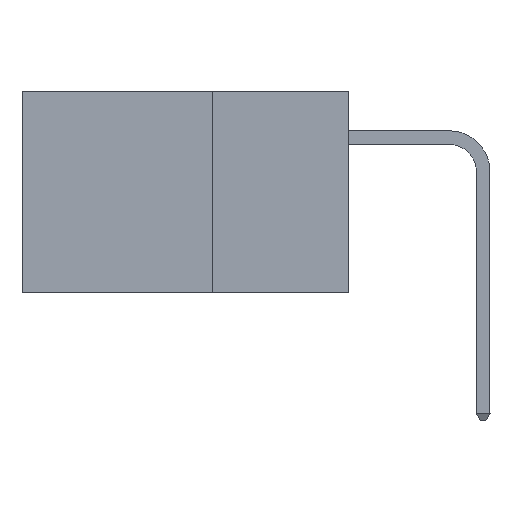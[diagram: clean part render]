
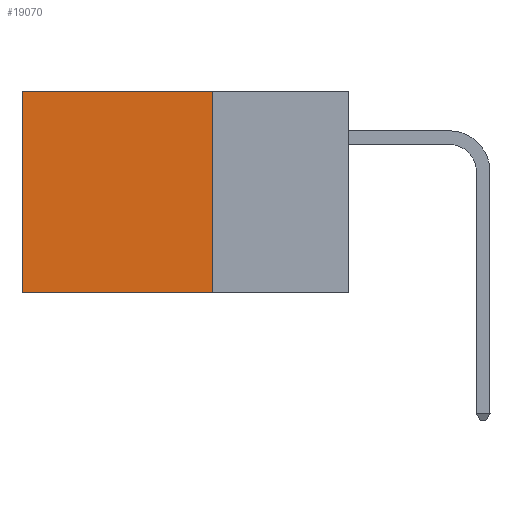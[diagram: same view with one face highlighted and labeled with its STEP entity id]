
A CAD part, left-side view. The second image highlights one B-rep face of the part: STEP entity #19070.
In plain terms, the highlighted planar face has unit normal (-1, 0, 0).
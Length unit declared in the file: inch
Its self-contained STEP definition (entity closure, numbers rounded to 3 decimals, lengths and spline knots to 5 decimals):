
#576 = EDGE_CURVE ( 'NONE', #24592, #1277, #18987, .T. ) ;
#1277 = VERTEX_POINT ( 'NONE', #18272 ) ;
#1332 = ORIENTED_EDGE ( 'NONE', *, *, #10872, .F. ) ;
#1830 = CARTESIAN_POINT ( 'NONE',  ( 0.2875, 0.25, 0. ) ) ;
#2749 = CARTESIAN_POINT ( 'NONE',  ( 0.2875, 0.6, 0. ) ) ;
#3491 = LINE ( 'NONE', #5325, #19199 ) ;
#5055 = VECTOR ( 'NONE', #14273, 39.37008 ) ;
#5325 = CARTESIAN_POINT ( 'NONE',  ( 0.2875, 0.25, -0.37 ) ) ;
#5871 = AXIS2_PLACEMENT_3D ( 'NONE', #6018, #14268, #10321 ) ;
#6018 = CARTESIAN_POINT ( 'NONE',  ( 0.2875, 0.25, 0. ) ) ;
#6700 = EDGE_CURVE ( 'NONE', #17373, #1277, #3491, .T. ) ;
#7690 = VERTEX_POINT ( 'NONE', #10959 ) ;
#8806 = CARTESIAN_POINT ( 'NONE',  ( 0.2875, 0.25, -0.37 ) ) ;
#10049 = CARTESIAN_POINT ( 'NONE',  ( 0.2875, 0.6, 0. ) ) ;
#10321 = DIRECTION ( 'NONE',  ( 0., 0., -1. ) ) ;
#10474 = EDGE_CURVE ( 'NONE', #7690, #24592, #12975, .T. ) ;
#10872 = EDGE_CURVE ( 'NONE', #7690, #17373, #23862, .T. ) ;
#10943 = VECTOR ( 'NONE', #18874, 39.37008 ) ;
#10959 = CARTESIAN_POINT ( 'NONE',  ( 0.2875, 0.25, 0. ) ) ;
#12131 = EDGE_LOOP ( 'NONE', ( #19035, #12728, #1332, #13910 ) ) ;
#12728 = ORIENTED_EDGE ( 'NONE', *, *, #6700, .F. ) ;
#12975 = LINE ( 'NONE', #15085, #10943 ) ;
#13910 = ORIENTED_EDGE ( 'NONE', *, *, #10474, .T. ) ;
#14268 = DIRECTION ( 'NONE',  ( 1., 0., 0. ) ) ;
#14273 = DIRECTION ( 'NONE',  ( 0., 0., -1. ) ) ;
#15085 = CARTESIAN_POINT ( 'NONE',  ( 0.2875, 0.25, 0. ) ) ;
#17373 = VERTEX_POINT ( 'NONE', #8806 ) ;
#18272 = CARTESIAN_POINT ( 'NONE',  ( 0.2875, 0.6, -0.37 ) ) ;
#18727 = DIRECTION ( 'NONE',  ( 0., 0., -1. ) ) ;
#18874 = DIRECTION ( 'NONE',  ( 0., 1., 0. ) ) ;
#18987 = LINE ( 'NONE', #2749, #19183 ) ;
#19035 = ORIENTED_EDGE ( 'NONE', *, *, #576, .T. ) ;
#19070 = ADVANCED_FACE ( 'NONE', ( #22405 ), #20032, .F. ) ;
#19183 = VECTOR ( 'NONE', #18727, 39.37008 ) ;
#19199 = VECTOR ( 'NONE', #23419, 39.37008 ) ;
#20032 = PLANE ( 'NONE',  #5871 ) ;
#22405 = FACE_OUTER_BOUND ( 'NONE', #12131, .T. ) ;
#23419 = DIRECTION ( 'NONE',  ( 0., 1., 0. ) ) ;
#23862 = LINE ( 'NONE', #1830, #5055 ) ;
#24592 = VERTEX_POINT ( 'NONE', #10049 ) ;
